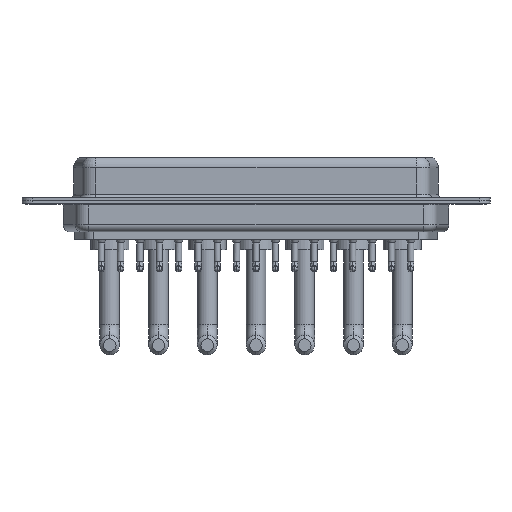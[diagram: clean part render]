
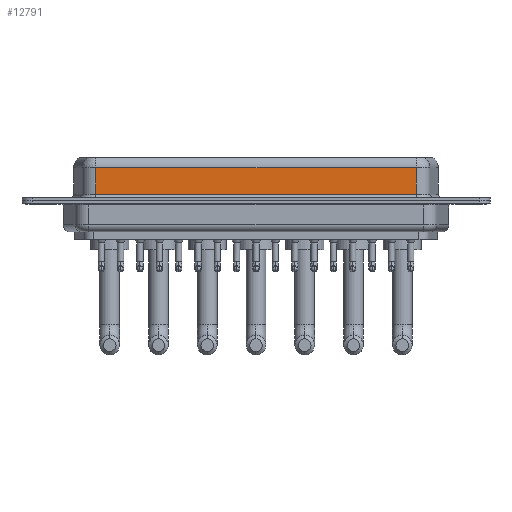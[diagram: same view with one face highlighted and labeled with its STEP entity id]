
A CAD part, front view. The second image highlights one B-rep face of the part: STEP entity #12791.
In plain terms, the highlighted planar face has unit normal (0, -1, 0).
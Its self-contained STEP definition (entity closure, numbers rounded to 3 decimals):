
#870 = FACE_OUTER_BOUND ( 'NONE', #14588, .T. ) ;
#943 = VERTEX_POINT ( 'NONE', #10452 ) ;
#1084 = CARTESIAN_POINT ( 'NONE',  ( 53.41, -5.375, 0.9 ) ) ;
#1158 = EDGE_CURVE ( 'NONE', #2902, #13231, #2102, .T. ) ;
#1535 = AXIS2_PLACEMENT_3D ( 'NONE', #11074, #17070, #9893 ) ;
#1919 = VECTOR ( 'NONE', #5779, 1000. ) ;
#2102 = LINE ( 'NONE', #3763, #16298 ) ;
#2902 = VERTEX_POINT ( 'NONE', #4568 ) ;
#3016 = ORIENTED_EDGE ( 'NONE', *, *, #14656, .T. ) ;
#3763 = CARTESIAN_POINT ( 'NONE',  ( 53.41, -5.375, 6.4 ) ) ;
#4568 = CARTESIAN_POINT ( 'NONE',  ( 53.41, -5.375, 4.65 ) ) ;
#5087 = ORIENTED_EDGE ( 'NONE', *, *, #6781, .T. ) ;
#5416 = ORIENTED_EDGE ( 'NONE', *, *, #5428, .T. ) ;
#5428 = EDGE_CURVE ( 'NONE', #15908, #13231, #14525, .T. ) ;
#5525 = CARTESIAN_POINT ( 'NONE',  ( 7.59, -5.375, 0.9 ) ) ;
#5779 = DIRECTION ( 'NONE',  ( 0., 0., -1. ) ) ;
#6223 = ORIENTED_EDGE ( 'NONE', *, *, #1158, .F. ) ;
#6781 = EDGE_CURVE ( 'NONE', #943, #15908, #16374, .T. ) ;
#8493 = VECTOR ( 'NONE', #14622, 1000. ) ;
#8566 = DIRECTION ( 'NONE',  ( -1., 0., 0. ) ) ;
#8918 = CARTESIAN_POINT ( 'NONE',  ( 7.59, -5.375, 6.4 ) ) ;
#9893 = DIRECTION ( 'NONE',  ( 0., 0., 1. ) ) ;
#10030 = LINE ( 'NONE', #15928, #14742 ) ;
#10452 = CARTESIAN_POINT ( 'NONE',  ( 7.59, -5.375, 4.65 ) ) ;
#11074 = CARTESIAN_POINT ( 'NONE',  ( 53.41, -5.375, 6.4 ) ) ;
#11129 = DIRECTION ( 'NONE',  ( 0., 0., -1. ) ) ;
#12542 = PLANE ( 'NONE',  #1535 ) ;
#12791 = ADVANCED_FACE ( 'NONE', ( #870 ), #12542, .F. ) ;
#13231 = VERTEX_POINT ( 'NONE', #14005 ) ;
#14005 = CARTESIAN_POINT ( 'NONE',  ( 53.41, -5.375, 0.9 ) ) ;
#14525 = LINE ( 'NONE', #1084, #8493 ) ;
#14588 = EDGE_LOOP ( 'NONE', ( #6223, #3016, #5087, #5416 ) ) ;
#14622 = DIRECTION ( 'NONE',  ( 1., 0., 0. ) ) ;
#14656 = EDGE_CURVE ( 'NONE', #2902, #943, #10030, .T. ) ;
#14742 = VECTOR ( 'NONE', #8566, 1000. ) ;
#15908 = VERTEX_POINT ( 'NONE', #5525 ) ;
#15928 = CARTESIAN_POINT ( 'NONE',  ( 53.41, -5.375, 4.65 ) ) ;
#16298 = VECTOR ( 'NONE', #11129, 1000. ) ;
#16374 = LINE ( 'NONE', #8918, #1919 ) ;
#17070 = DIRECTION ( 'NONE',  ( 0., 1., 0. ) ) ;
